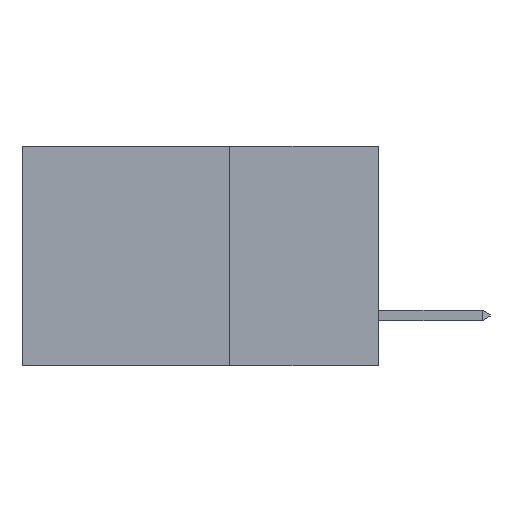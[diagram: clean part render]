
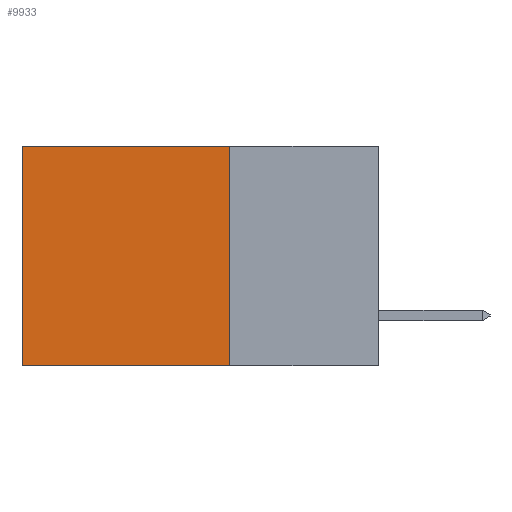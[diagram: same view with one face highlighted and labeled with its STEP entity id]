
A CAD part, left-side view. The second image highlights one B-rep face of the part: STEP entity #9933.
In plain terms, the highlighted planar face has unit normal (-1, 0, 0).
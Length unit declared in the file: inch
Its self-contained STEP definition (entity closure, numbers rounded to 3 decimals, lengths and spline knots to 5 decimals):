
#922 = LINE ( 'NONE', #5043, #7225 ) ;
#1125 = DIRECTION ( 'NONE',  ( 0., 0., -1. ) ) ;
#1191 = AXIS2_PLACEMENT_3D ( 'NONE', #10905, #12197, #4576 ) ;
#1313 = VERTEX_POINT ( 'NONE', #13730 ) ;
#1541 = VERTEX_POINT ( 'NONE', #9687 ) ;
#3360 = EDGE_CURVE ( 'NONE', #5875, #1541, #922, .T. ) ;
#4158 = DIRECTION ( 'NONE',  ( 0., 1., 0. ) ) ;
#4576 = DIRECTION ( 'NONE',  ( 0., 0., -1. ) ) ;
#4777 = LINE ( 'NONE', #6115, #11148 ) ;
#4830 = CARTESIAN_POINT ( 'NONE',  ( 0.2615, 0.25, 0. ) ) ;
#5043 = CARTESIAN_POINT ( 'NONE',  ( 0.2615, 0.6, -0.37 ) ) ;
#5424 = EDGE_CURVE ( 'NONE', #1313, #5875, #9496, .T. ) ;
#5544 = FACE_OUTER_BOUND ( 'NONE', #14688, .T. ) ;
#5691 = VECTOR ( 'NONE', #6100, 39.37008 ) ;
#5875 = VERTEX_POINT ( 'NONE', #9432 ) ;
#6100 = DIRECTION ( 'NONE',  ( 0., 1., 0. ) ) ;
#6115 = CARTESIAN_POINT ( 'NONE',  ( 0.2615, 0.25, -0.37 ) ) ;
#6619 = ORIENTED_EDGE ( 'NONE', *, *, #14587, .F. ) ;
#6822 = VECTOR ( 'NONE', #4158, 39.37008 ) ;
#7225 = VECTOR ( 'NONE', #13946, 39.37008 ) ;
#9404 = ORIENTED_EDGE ( 'NONE', *, *, #3360, .T. ) ;
#9432 = CARTESIAN_POINT ( 'NONE',  ( 0.2615, 0.6, 0. ) ) ;
#9496 = LINE ( 'NONE', #4830, #5691 ) ;
#9637 = PLANE ( 'NONE',  #1191 ) ;
#9687 = CARTESIAN_POINT ( 'NONE',  ( 0.2615, 0.6, -0.37 ) ) ;
#9802 = ORIENTED_EDGE ( 'NONE', *, *, #9977, .F. ) ;
#9933 = ADVANCED_FACE ( 'NONE', ( #5544 ), #9637, .F. ) ;
#9977 = EDGE_CURVE ( 'NONE', #1313, #11990, #4777, .T. ) ;
#10225 = LINE ( 'NONE', #10454, #6822 ) ;
#10454 = CARTESIAN_POINT ( 'NONE',  ( 0.2615, 0.25, -0.37 ) ) ;
#10905 = CARTESIAN_POINT ( 'NONE',  ( 0.2615, 0.25, -0.37 ) ) ;
#11148 = VECTOR ( 'NONE', #1125, 39.37008 ) ;
#11990 = VERTEX_POINT ( 'NONE', #14852 ) ;
#12197 = DIRECTION ( 'NONE',  ( 1., 0., 0. ) ) ;
#12892 = ORIENTED_EDGE ( 'NONE', *, *, #5424, .T. ) ;
#13730 = CARTESIAN_POINT ( 'NONE',  ( 0.2615, 0.25, 0. ) ) ;
#13946 = DIRECTION ( 'NONE',  ( 0., 0., -1. ) ) ;
#14587 = EDGE_CURVE ( 'NONE', #11990, #1541, #10225, .T. ) ;
#14688 = EDGE_LOOP ( 'NONE', ( #9404, #6619, #9802, #12892 ) ) ;
#14852 = CARTESIAN_POINT ( 'NONE',  ( 0.2615, 0.25, -0.37 ) ) ;
